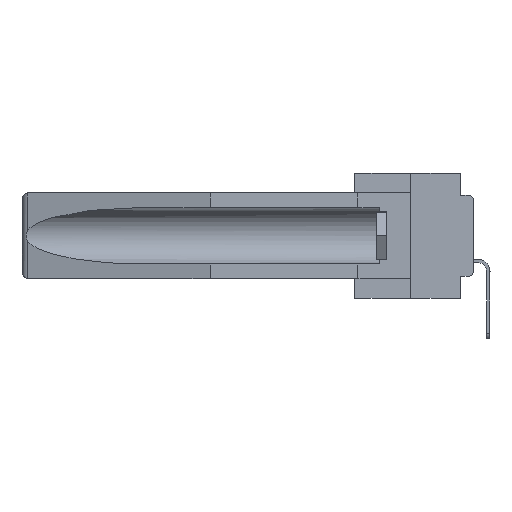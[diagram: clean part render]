
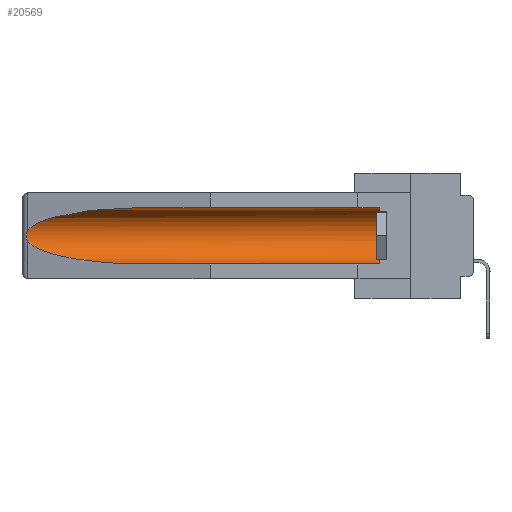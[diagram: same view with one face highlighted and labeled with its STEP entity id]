
A CAD part, left-side view. The second image highlights one B-rep face of the part: STEP entity #20569.
In plain terms, the highlighted cylindrical face has radius 2.857 mm (diameter 5.715 mm), a partial arc.
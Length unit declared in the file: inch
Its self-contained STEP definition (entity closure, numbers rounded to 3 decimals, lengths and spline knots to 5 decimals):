
#889 = VECTOR ( 'NONE', #8431, 39.37008 ) ;
#1429 = CYLINDRICAL_SURFACE ( 'NONE', #21985, 0.1125 ) ;
#2516 = EDGE_CURVE ( 'NONE', #25596, #16104, #7509, .T. ) ;
#2694 = VERTEX_POINT ( 'NONE', #3956 ) ;
#3100 = VERTEX_POINT ( 'NONE', #21353 ) ;
#3863 = ORIENTED_EDGE ( 'NONE', *, *, #7820, .T. ) ;
#3956 = CARTESIAN_POINT ( 'NONE',  ( 0.155, 1.07973, -0.284 ) ) ;
#4432 = CARTESIAN_POINT ( 'NONE',  ( 0.26654, 1.53092, -0.15636 ) ) ;
#6229 = FACE_OUTER_BOUND ( 'NONE', #7239, .T. ) ;
#6533 = CARTESIAN_POINT ( 'NONE',  ( 0.155, -0.30754, -0.1715 ) ) ;
#6621 = CARTESIAN_POINT ( 'NONE',  ( 0.26597, 1.5296, -0.19026 ) ) ;
#7017 = ORIENTED_EDGE ( 'NONE', *, *, #27260, .T. ) ;
#7239 = EDGE_LOOP ( 'NONE', ( #11771, #7017, #21232, #29277, #28760, #3863 ) ) ;
#7509 = CIRCLE ( 'NONE', #29663, 0.1125 ) ;
#7820 = EDGE_CURVE ( 'NONE', #16104, #3100, #22007, .T. ) ;
#8431 = DIRECTION ( 'NONE',  ( 0., 1., 0. ) ) ;
#8559 = CARTESIAN_POINT ( 'NONE',  ( 0.155, 1.07973, -0.284 ) ) ;
#8628 = CARTESIAN_POINT ( 'NONE',  ( 0.2675, 1.53308, -0.17534 ) ) ;
#8693 = DIRECTION ( 'NONE',  ( 0., 0., 1. ) ) ;
#9299 = CARTESIAN_POINT ( 'NONE',  ( 0.26537, 1.52718, -0.14972 ) ) ;
#11351 = CARTESIAN_POINT ( 'NONE',  ( 0.26537, 1.52718, -0.14972 ) ) ;
#11391 = CARTESIAN_POINT ( 'NONE',  ( 0.155, 0.126, -0.284 ) ) ;
#11771 = ORIENTED_EDGE ( 'NONE', *, *, #13674, .T. ) ;
#13488 = CARTESIAN_POINT ( 'NONE',  ( 0.155, -0.30754, -0.284 ) ) ;
#13674 = EDGE_CURVE ( 'NONE', #3100, #18082, #15415, .T. ) ;
#13809 = CARTESIAN_POINT ( 'NONE',  ( 0.2673, 1.5327, -0.16383 ) ) ;
#15277 = DIRECTION ( 'NONE',  ( 0., 0., 1. ) ) ;
#15415 =( BOUNDED_CURVE ( )  B_SPLINE_CURVE ( 3, ( #25647, #20560, #29956, #9299 ),
 .UNSPECIFIED., .F., .F. ) 
 B_SPLINE_CURVE_WITH_KNOTS ( ( 4, 4 ),
 ( 4.71239, 6.08839 ),
 .UNSPECIFIED. ) 
 CURVE ( )  GEOMETRIC_REPRESENTATION_ITEM ( )  RATIONAL_B_SPLINE_CURVE ( ( 1., 0.848, 0.848, 1. ) ) 
 REPRESENTATION_ITEM ( '' )  );
#16016 = CARTESIAN_POINT ( 'NONE',  ( 0.2675, 1.53308, -0.16763 ) ) ;
#16104 = VERTEX_POINT ( 'NONE', #29388 ) ;
#16283 = EDGE_CURVE ( 'NONE', #25596, #2694, #22917, .T. ) ;
#16402 =( BOUNDED_CURVE ( )  B_SPLINE_CURVE ( 3, ( #24626, #29671, #20434, #8559 ),
 .UNSPECIFIED., .F., .F. ) 
 B_SPLINE_CURVE_WITH_KNOTS ( ( 4, 4 ),
 ( 0.1948, 1.5708 ),
 .UNSPECIFIED. ) 
 CURVE ( )  GEOMETRIC_REPRESENTATION_ITEM ( )  RATIONAL_B_SPLINE_CURVE ( ( 1., 0.848, 0.848, 1. ) ) 
 REPRESENTATION_ITEM ( '' )  );
#17751 = CARTESIAN_POINT ( 'NONE',  ( 0.155, 0.126, -0.1715 ) ) ;
#18082 = VERTEX_POINT ( 'NONE', #18723 ) ;
#18723 = CARTESIAN_POINT ( 'NONE',  ( 0.26537, 1.52718, -0.14972 ) ) ;
#19078 = DIRECTION ( 'NONE',  ( 0., 1., 0. ) ) ;
#19719 = CARTESIAN_POINT ( 'NONE',  ( 0.155, -0.30754, -0.059 ) ) ;
#19969 = B_SPLINE_CURVE_WITH_KNOTS ( 'NONE', 3,
 ( #11351, #20774, #4432, #13809, #16016, #8628, #22510, #22363, #6621, #22967 ),
 .UNSPECIFIED., .F., .F.,
 ( 4, 2, 2, 2, 4 ),
 ( 0., 0.00029, 0.00058, 0.00087, 0.00117 ),
 .UNSPECIFIED. ) ;
#20434 = CARTESIAN_POINT ( 'NONE',  ( 0.21114, 1.30732, -0.284 ) ) ;
#20560 = CARTESIAN_POINT ( 'NONE',  ( 0.21114, 1.30732, -0.059 ) ) ;
#20569 = ADVANCED_FACE ( 'NONE', ( #6229 ), #1429, .F. ) ;
#20774 = CARTESIAN_POINT ( 'NONE',  ( 0.26597, 1.52961, -0.15275 ) ) ;
#21232 = ORIENTED_EDGE ( 'NONE', *, *, #28203, .T. ) ;
#21353 = CARTESIAN_POINT ( 'NONE',  ( 0.155, 1.07973, -0.059 ) ) ;
#21943 = CARTESIAN_POINT ( 'NONE',  ( 0.26537, 1.52718, -0.19328 ) ) ;
#21985 = AXIS2_PLACEMENT_3D ( 'NONE', #6533, #25198, #8693 ) ;
#22007 = LINE ( 'NONE', #19719, #25096 ) ;
#22363 = CARTESIAN_POINT ( 'NONE',  ( 0.26655, 1.53094, -0.18657 ) ) ;
#22510 = CARTESIAN_POINT ( 'NONE',  ( 0.2673, 1.53269, -0.17917 ) ) ;
#22917 = LINE ( 'NONE', #13488, #889 ) ;
#22967 = CARTESIAN_POINT ( 'NONE',  ( 0.26537, 1.52718, -0.19328 ) ) ;
#23679 = VERTEX_POINT ( 'NONE', #21943 ) ;
#24626 = CARTESIAN_POINT ( 'NONE',  ( 0.26537, 1.52718, -0.19328 ) ) ;
#25096 = VECTOR ( 'NONE', #19078, 39.37008 ) ;
#25198 = DIRECTION ( 'NONE',  ( 0., 1., 0. ) ) ;
#25596 = VERTEX_POINT ( 'NONE', #11391 ) ;
#25647 = CARTESIAN_POINT ( 'NONE',  ( 0.155, 1.07973, -0.059 ) ) ;
#27135 = DIRECTION ( 'NONE',  ( 0., -1., 0. ) ) ;
#27260 = EDGE_CURVE ( 'NONE', #18082, #23679, #19969, .T. ) ;
#28203 = EDGE_CURVE ( 'NONE', #23679, #2694, #16402, .T. ) ;
#28760 = ORIENTED_EDGE ( 'NONE', *, *, #2516, .T. ) ;
#29277 = ORIENTED_EDGE ( 'NONE', *, *, #16283, .F. ) ;
#29388 = CARTESIAN_POINT ( 'NONE',  ( 0.155, 0.126, -0.059 ) ) ;
#29663 = AXIS2_PLACEMENT_3D ( 'NONE', #17751, #27135, #15277 ) ;
#29671 = CARTESIAN_POINT ( 'NONE',  ( 0.25451, 1.48313, -0.24835 ) ) ;
#29956 = CARTESIAN_POINT ( 'NONE',  ( 0.25451, 1.48313, -0.09465 ) ) ;
